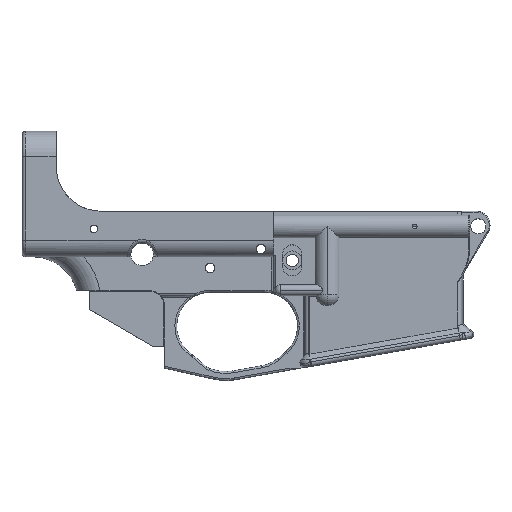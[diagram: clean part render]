
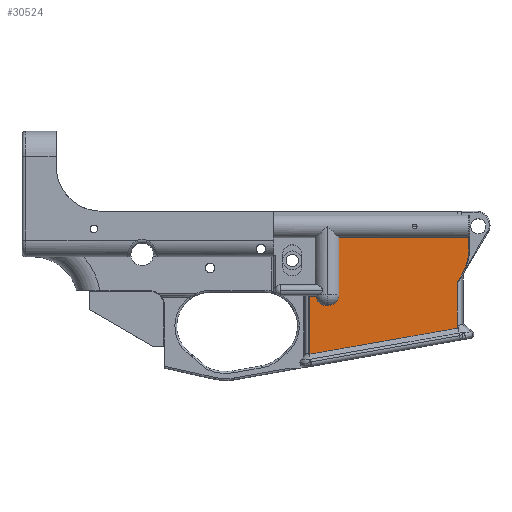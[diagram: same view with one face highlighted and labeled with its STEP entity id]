
A CAD part, top view. The second image highlights one B-rep face of the part: STEP entity #30524.
In plain terms, the highlighted planar face has unit normal (0, 0, 1).
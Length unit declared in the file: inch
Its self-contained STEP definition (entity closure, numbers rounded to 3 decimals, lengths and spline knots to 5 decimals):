
#76 = CARTESIAN_POINT ( 'NONE',  ( -0.34789, -1.68872, 0.5925 ) ) ;
#89 = CARTESIAN_POINT ( 'NONE',  ( -2.8015, -2.12136, 0.5925 ) ) ;
#170 = CARTESIAN_POINT ( 'NONE',  ( -2.8015, -1.1595, 0.5925 ) ) ;
#238 = CARTESIAN_POINT ( 'NONE',  ( -0.155, -0.35559, 0.5925 ) ) ;
#246 = CARTESIAN_POINT ( 'NONE',  ( -0.28406, -0.82412, 0.5925 ) ) ;
#329 = CARTESIAN_POINT ( 'NONE',  ( -0.34789, -0.93121, 0.5925 ) ) ;
#356 = CARTESIAN_POINT ( 'NONE',  ( -0.155, -0.18642, 0.5925 ) ) ;
#3179 = EDGE_LOOP ( 'NONE', ( #53097, #53098, #53099, #53100, #53101, #53102, #53103, #53104, #53105, #53106, #53107 ) ) ;
#3566 = VERTEX_POINT ( 'NONE', #76 ) ;
#3567 = VERTEX_POINT ( 'NONE', #89 ) ;
#6512 = CARTESIAN_POINT ( 'NONE',  ( -1.07, -0.35559, 0.5925 ) ) ;
#6514 = PLANE ( 'NONE',  #40084 ) ;
#6516 = DIRECTION ( 'NONE',  ( 0., 0., 1. ) ) ;
#6517 = DIRECTION ( 'NONE',  ( 1., 0., 0. ) ) ;
#7167 = FACE_OUTER_BOUND ( 'NONE', #3179, .T. ) ;
#13479 = VERTEX_POINT ( 'NONE', #170 ) ;
#13493 = VERTEX_POINT ( 'NONE', #329 ) ;
#13503 = VERTEX_POINT ( 'NONE', #246 ) ;
#13507 = VERTEX_POINT ( 'NONE', #238 ) ;
#13510 = VERTEX_POINT ( 'NONE', #356 ) ;
#14868 = VERTEX_POINT ( 'NONE', #45260 ) ;
#14879 = VERTEX_POINT ( 'NONE', #45363 ) ;
#17422 = CARTESIAN_POINT ( 'NONE',  ( -2.31133, -1.1333, 0.5925 ) ) ;
#17424 = CARTESIAN_POINT ( 'NONE',  ( -2.31133, -0.18642, 0.5925 ) ) ;
#29434 = CARTESIAN_POINT ( 'NONE',  ( -2.52537, -1.31289, 0.5925 ) ) ;
#29438 = CARTESIAN_POINT ( 'NONE',  ( -2.503, -1.31289, 0.5925 ) ) ;
#29445 = CARTESIAN_POINT ( 'NONE',  ( -2.5472, -1.30974, 0.5925 ) ) ;
#29446 = CARTESIAN_POINT ( 'NONE',  ( -2.57902, -1.29953, 0.5925 ) ) ;
#29447 = CARTESIAN_POINT ( 'NONE',  ( -2.58938, -1.2952, 0.5925 ) ) ;
#29448 = CARTESIAN_POINT ( 'NONE',  ( -2.60894, -1.28488, 0.5925 ) ) ;
#29449 = CARTESIAN_POINT ( 'NONE',  ( -2.61824, -1.27886, 0.5925 ) ) ;
#29450 = CARTESIAN_POINT ( 'NONE',  ( -2.63582, -1.26502, 0.5925 ) ) ;
#29451 = CARTESIAN_POINT ( 'NONE',  ( -2.6439, -1.25733, 0.5925 ) ) ;
#29452 = CARTESIAN_POINT ( 'NONE',  ( -2.65843, -1.24069, 0.5925 ) ) ;
#29453 = CARTESIAN_POINT ( 'NONE',  ( -2.66493, -1.23168, 0.5925 ) ) ;
#29454 = CARTESIAN_POINT ( 'NONE',  ( -2.67625, -1.21233, 0.5925 ) ) ;
#29455 = CARTESIAN_POINT ( 'NONE',  ( -2.68091, -1.20228, 0.5925 ) ) ;
#29456 = CARTESIAN_POINT ( 'NONE',  ( -2.68829, -1.18143, 0.5925 ) ) ;
#29457 = CARTESIAN_POINT ( 'NONE',  ( -2.69103, -1.17052, 0.5925 ) ) ;
#29458 = CARTESIAN_POINT ( 'NONE',  ( -2.6927, -1.1595, 0.5925 ) ) ;
#30524 = ADVANCED_FACE ( 'NONE', ( #7167 ), #6514, .T. ) ;
#40084 = AXIS2_PLACEMENT_3D ( 'NONE', #6512, #6516, #6517 ) ;
#40604 = VERTEX_POINT ( 'NONE', #17422 ) ;
#40606 = VERTEX_POINT ( 'NONE', #17424 ) ;
#41868 = EDGE_CURVE ( 'NONE', #14879, #13479, #44118, .T. ) ;
#41869 = EDGE_CURVE ( 'NONE', #13479, #3567, #44131, .T. ) ;
#41870 = EDGE_CURVE ( 'NONE', #3566, #13493, #44139, .T. ) ;
#41871 = EDGE_CURVE ( 'NONE', #13493, #13503, #44144, .T. ) ;
#41872 = EDGE_CURVE ( 'NONE', #13503, #13507, #44148, .T. ) ;
#41873 = EDGE_CURVE ( 'NONE', #13507, #13510, #44152, .T. ) ;
#41874 = EDGE_CURVE ( 'NONE', #13510, #40606, #44154, .T. ) ;
#42305 = EDGE_CURVE ( 'NONE', #3566, #3567, #44978, .T. ) ;
#42460 = EDGE_CURVE ( 'NONE', #40604, #14868, #49408, .T. ) ;
#42462 = EDGE_CURVE ( 'NONE', #40606, #40604, #45041, .T. ) ;
#43280 = CARTESIAN_POINT ( 'NONE',  ( -1.07, -1.1595, 0.5925 ) ) ;
#43297 = CARTESIAN_POINT ( 'NONE',  ( -2.8015, -2.12449, 0.5925 ) ) ;
#43301 = DIRECTION ( 'NONE',  ( 0., 1., 0. ) ) ;
#43303 = DIRECTION ( 'NONE',  ( -1., 0., 0. ) ) ;
#43304 = CARTESIAN_POINT ( 'NONE',  ( -0.155, -0.17959, 0.5925 ) ) ;
#43305 = DIRECTION ( 'NONE',  ( 0., -1., 0. ) ) ;
#43306 = CARTESIAN_POINT ( 'NONE',  ( -0.34789, -0.93396, 0.5925 ) ) ;
#43307 = DIRECTION ( 'NONE',  ( 0., 1., 0. ) ) ;
#43308 = CARTESIAN_POINT ( 'NONE',  ( -0.28406, -0.82412, 0.5925 ) ) ;
#43309 = DIRECTION ( 'NONE',  ( 0.512, 0.859, 0. ) ) ;
#43312 = CARTESIAN_POINT ( 'NONE',  ( -1.07, -0.35559, 0.5925 ) ) ;
#43313 = DIRECTION ( 'NONE',  ( 0., 0., 1. ) ) ;
#43314 = DIRECTION ( 'NONE',  ( 1., 0., 0. ) ) ;
#43315 = CARTESIAN_POINT ( 'NONE',  ( -2.31133, -0.18642, 0.5925 ) ) ;
#43316 = DIRECTION ( 'NONE',  ( -1., 0., 0. ) ) ;
#44118 = LINE ( 'NONE', #43280, #44137 ) ;
#44131 = LINE ( 'NONE', #43297, #44141 ) ;
#44137 = VECTOR ( 'NONE', #43303, 39.37008 ) ;
#44139 = LINE ( 'NONE', #43306, #44146 ) ;
#44141 = VECTOR ( 'NONE', #43305, 39.37008 ) ;
#44144 = LINE ( 'NONE', #43308, #44150 ) ;
#44146 = VECTOR ( 'NONE', #43307, 39.37008 ) ;
#44148 = CIRCLE ( 'NONE', #45322, 0.915 ) ;
#44150 = VECTOR ( 'NONE', #43309, 39.37008 ) ;
#44152 = LINE ( 'NONE', #43304, #44157 ) ;
#44154 = LINE ( 'NONE', #43315, #44160 ) ;
#44157 = VECTOR ( 'NONE', #43301, 39.37008 ) ;
#44160 = VECTOR ( 'NONE', #43316, 39.37008 ) ;
#44978 = LINE ( 'NONE', #47547, #44979 ) ;
#44979 = VECTOR ( 'NONE', #47548, 39.37008 ) ;
#45041 = LINE ( 'NONE', #48504, #45044 ) ;
#45044 = VECTOR ( 'NONE', #48475, 39.37008 ) ;
#45260 = CARTESIAN_POINT ( 'NONE',  ( -2.503, -1.31289, 0.5925 ) ) ;
#45322 = AXIS2_PLACEMENT_3D ( 'NONE', #43312, #43313, #43314 ) ;
#45363 = CARTESIAN_POINT ( 'NONE',  ( -2.6927, -1.1595, 0.5925 ) ) ;
#47547 = CARTESIAN_POINT ( 'NONE',  ( 0.2783, -1.57831, 0.5925 ) ) ;
#47548 = DIRECTION ( 'NONE',  ( -0.985, -0.174, 0. ) ) ;
#48475 = DIRECTION ( 'NONE',  ( 0., -1., 0. ) ) ;
#48479 = CARTESIAN_POINT ( 'NONE',  ( -2.31133, -1.13941, 0.5925 ) ) ;
#48480 = CARTESIAN_POINT ( 'NONE',  ( -2.31133, -1.1333, 0.5925 ) ) ;
#48484 = CARTESIAN_POINT ( 'NONE',  ( -2.31166, -1.14558, 0.5925 ) ) ;
#48485 = CARTESIAN_POINT ( 'NONE',  ( -2.31293, -1.15771, 0.5925 ) ) ;
#48486 = CARTESIAN_POINT ( 'NONE',  ( -2.31389, -1.16371, 0.5925 ) ) ;
#48487 = CARTESIAN_POINT ( 'NONE',  ( -2.31766, -1.18151, 0.5925 ) ) ;
#48488 = CARTESIAN_POINT ( 'NONE',  ( -2.32143, -1.1932, 0.5925 ) ) ;
#48489 = CARTESIAN_POINT ( 'NONE',  ( -2.33135, -1.21559, 0.5925 ) ) ;
#48490 = CARTESIAN_POINT ( 'NONE',  ( -2.3374, -1.22611, 0.5925 ) ) ;
#48491 = CARTESIAN_POINT ( 'NONE',  ( -2.3516, -1.24585, 0.5925 ) ) ;
#48492 = CARTESIAN_POINT ( 'NONE',  ( -2.35985, -1.25511, 0.5925 ) ) ;
#48493 = CARTESIAN_POINT ( 'NONE',  ( -2.37778, -1.27152, 0.5925 ) ) ;
#48494 = CARTESIAN_POINT ( 'NONE',  ( -2.38752, -1.27878, 0.5925 ) ) ;
#48495 = CARTESIAN_POINT ( 'NONE',  ( -2.40855, -1.29139, 0.5925 ) ) ;
#48496 = CARTESIAN_POINT ( 'NONE',  ( -2.41963, -1.29659, 0.5925 ) ) ;
#48497 = CARTESIAN_POINT ( 'NONE',  ( -2.44247, -1.30483, 0.5925 ) ) ;
#48498 = CARTESIAN_POINT ( 'NONE',  ( -2.45438, -1.30789, 0.5925 ) ) ;
#48499 = CARTESIAN_POINT ( 'NONE',  ( -2.47853, -1.31191, 0.5925 ) ) ;
#48500 = CARTESIAN_POINT ( 'NONE',  ( -2.49075, -1.31289, 0.5925 ) ) ;
#48501 = CARTESIAN_POINT ( 'NONE',  ( -2.503, -1.31289, 0.5925 ) ) ;
#48504 = CARTESIAN_POINT ( 'NONE',  ( -2.31133, -1.32481, 0.5925 ) ) ;
#49408 = B_SPLINE_CURVE_WITH_KNOTS ( 'NONE', 3,
 ( #48480, #48479, #48484, #48485, #48486, #48487, #48488, #48489, #48490, #48491, #48492, #48493, #48494, #48495, #48496, #48497, #48498, #48499, #48500, #48501 ),
 .UNSPECIFIED., .F., .F.,
 ( 4, 2, 2, 2, 2, 2, 2, 2, 2, 4 ),
 ( 0.02216, 0.02262, 0.02308, 0.024, 0.02493, 0.02585, 0.02677, 0.02769, 0.02861, 0.02953 ),
 .UNSPECIFIED. ) ;
#49615 = B_SPLINE_CURVE_WITH_KNOTS ( 'NONE', 3,
 ( #29438, #29434, #29445, #29446, #29447, #29448, #29449, #29450, #29451, #29452, #29453, #29454, #29455, #29456, #29457, #29458 ),
 .UNSPECIFIED., .F., .F.,
 ( 4, 2, 2, 2, 2, 2, 2, 4 ),
 ( 0.00002, 0.0017, 0.00254, 0.00338, 0.00422, 0.00506, 0.0059, 0.00674 ),
 .UNSPECIFIED. ) ;
#52462 = EDGE_CURVE ( 'NONE', #14868, #14879, #49615, .T. ) ;
#53097 = ORIENTED_EDGE ( 'NONE', *, *, #41868, .T. ) ;
#53098 = ORIENTED_EDGE ( 'NONE', *, *, #41869, .T. ) ;
#53099 = ORIENTED_EDGE ( 'NONE', *, *, #42305, .F. ) ;
#53100 = ORIENTED_EDGE ( 'NONE', *, *, #41870, .T. ) ;
#53101 = ORIENTED_EDGE ( 'NONE', *, *, #41871, .T. ) ;
#53102 = ORIENTED_EDGE ( 'NONE', *, *, #41872, .T. ) ;
#53103 = ORIENTED_EDGE ( 'NONE', *, *, #41873, .T. ) ;
#53104 = ORIENTED_EDGE ( 'NONE', *, *, #41874, .T. ) ;
#53105 = ORIENTED_EDGE ( 'NONE', *, *, #42462, .T. ) ;
#53106 = ORIENTED_EDGE ( 'NONE', *, *, #42460, .T. ) ;
#53107 = ORIENTED_EDGE ( 'NONE', *, *, #52462, .T. ) ;
